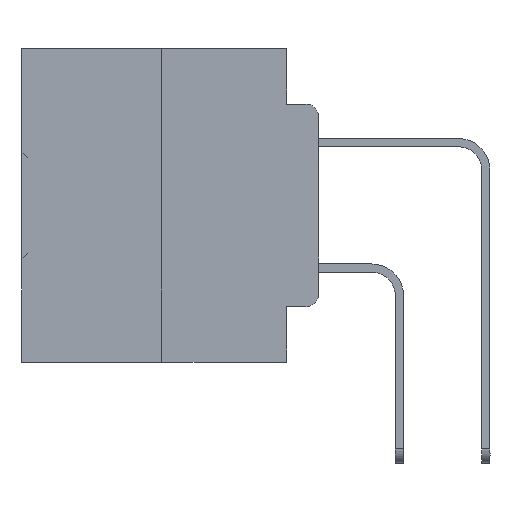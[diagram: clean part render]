
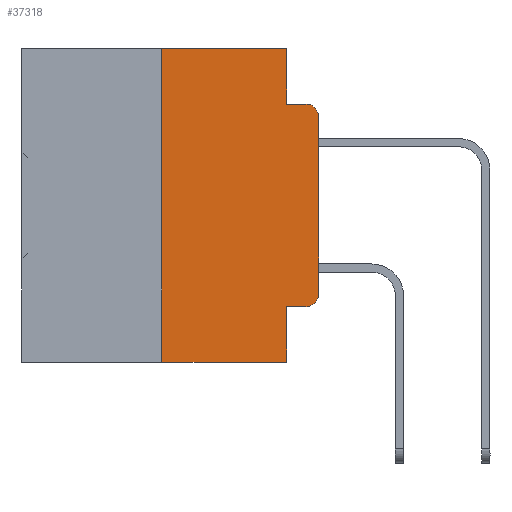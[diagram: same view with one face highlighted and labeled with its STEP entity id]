
A CAD part, left-side view. The second image highlights one B-rep face of the part: STEP entity #37318.
In plain terms, the highlighted planar face has unit normal (-1, 0, 0).
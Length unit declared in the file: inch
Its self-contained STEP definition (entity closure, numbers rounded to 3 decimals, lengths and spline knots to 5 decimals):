
#82 = VECTOR ( 'NONE', #9847, 39.37008 ) ;
#551 = ORIENTED_EDGE ( 'NONE', *, *, #11898, .T. ) ;
#628 = EDGE_CURVE ( 'NONE', #20644, #21502, #16890, .T. ) ;
#808 = CARTESIAN_POINT ( 'NONE',  ( 0., 0.02, -0.1085 ) ) ;
#951 = LINE ( 'NONE', #18273, #17860 ) ;
#1814 = DIRECTION ( 'NONE',  ( 1., 0., 0. ) ) ;
#1868 = DIRECTION ( 'NONE',  ( -1., 0., 0. ) ) ;
#1884 = ORIENTED_EDGE ( 'NONE', *, *, #18203, .F. ) ;
#2410 = CARTESIAN_POINT ( 'NONE',  ( 0., 0.051, -0.0885 ) ) ;
#2689 = CARTESIAN_POINT ( 'NONE',  ( 0., 0., -0.1085 ) ) ;
#2822 = VERTEX_POINT ( 'NONE', #36640 ) ;
#3727 = DIRECTION ( 'NONE',  ( 0., 0., 1. ) ) ;
#3755 = ORIENTED_EDGE ( 'NONE', *, *, #29755, .T. ) ;
#4560 = CIRCLE ( 'NONE', #31012, 0.02 ) ;
#5077 = PLANE ( 'NONE',  #7299 ) ;
#5140 = VERTEX_POINT ( 'NONE', #25508 ) ;
#5277 = CARTESIAN_POINT ( 'NONE',  ( 0., 0.25, 0. ) ) ;
#5418 = CARTESIAN_POINT ( 'NONE',  ( 0., 0.051, -0.5 ) ) ;
#6315 = DIRECTION ( 'NONE',  ( 0., 0., 1. ) ) ;
#6320 = EDGE_CURVE ( 'NONE', #5140, #35433, #21499, .T. ) ;
#6361 = VERTEX_POINT ( 'NONE', #36731 ) ;
#7162 = CARTESIAN_POINT ( 'NONE',  ( 0., 0., -0.3915 ) ) ;
#7299 = AXIS2_PLACEMENT_3D ( 'NONE', #22225, #1814, #22422 ) ;
#8712 = LINE ( 'NONE', #11243, #31086 ) ;
#9847 = DIRECTION ( 'NONE',  ( 0., 0., -1. ) ) ;
#10690 = ORIENTED_EDGE ( 'NONE', *, *, #628, .F. ) ;
#11243 = CARTESIAN_POINT ( 'NONE',  ( 0., 0.051, 0. ) ) ;
#11898 = EDGE_CURVE ( 'NONE', #6361, #26939, #4560, .T. ) ;
#11979 = EDGE_LOOP ( 'NONE', ( #26717, #3755, #10690, #24689, #18427, #1884, #12658, #35704, #31187, #551 ) ) ;
#12164 = LINE ( 'NONE', #30253, #82 ) ;
#12210 = CARTESIAN_POINT ( 'NONE',  ( 0., 0., 0. ) ) ;
#12476 = VECTOR ( 'NONE', #3727, 39.37008 ) ;
#12658 = ORIENTED_EDGE ( 'NONE', *, *, #6320, .T. ) ;
#14358 = CIRCLE ( 'NONE', #14960, 0.02 ) ;
#14960 = AXIS2_PLACEMENT_3D ( 'NONE', #808, #15659, #27743 ) ;
#15659 = DIRECTION ( 'NONE',  ( -1., 0., 0. ) ) ;
#15766 = DIRECTION ( 'NONE',  ( 0., -1., 0. ) ) ;
#16890 = LINE ( 'NONE', #2410, #23775 ) ;
#17860 = VECTOR ( 'NONE', #6315, 39.37008 ) ;
#17915 = CARTESIAN_POINT ( 'NONE',  ( 0., 0.473, 0. ) ) ;
#17986 = LINE ( 'NONE', #12210, #12476 ) ;
#18203 = EDGE_CURVE ( 'NONE', #5140, #37351, #951, .T. ) ;
#18273 = CARTESIAN_POINT ( 'NONE',  ( 0., 0.25, 0. ) ) ;
#18427 = ORIENTED_EDGE ( 'NONE', *, *, #34308, .F. ) ;
#19069 = EDGE_CURVE ( 'NONE', #2822, #35433, #12164, .T. ) ;
#19721 = FACE_OUTER_BOUND ( 'NONE', #11979, .T. ) ;
#20644 = VERTEX_POINT ( 'NONE', #25969 ) ;
#21499 = LINE ( 'NONE', #30919, #33946 ) ;
#21502 = VERTEX_POINT ( 'NONE', #30156 ) ;
#21923 = EDGE_CURVE ( 'NONE', #26939, #25903, #17986, .T. ) ;
#22041 = LINE ( 'NONE', #28192, #34871 ) ;
#22225 = CARTESIAN_POINT ( 'NONE',  ( 0., 0.473, 0. ) ) ;
#22422 = DIRECTION ( 'NONE',  ( 0., 0., -1. ) ) ;
#22502 = VERTEX_POINT ( 'NONE', #35769 ) ;
#23028 = DIRECTION ( 'NONE',  ( 0., -1., 0. ) ) ;
#23354 = DIRECTION ( 'NONE',  ( 0., 0., -1. ) ) ;
#23775 = VECTOR ( 'NONE', #23028, 39.37008 ) ;
#24689 = ORIENTED_EDGE ( 'NONE', *, *, #33732, .F. ) ;
#25508 = CARTESIAN_POINT ( 'NONE',  ( 0., 0.25, -0.5 ) ) ;
#25903 = VERTEX_POINT ( 'NONE', #2689 ) ;
#25969 = CARTESIAN_POINT ( 'NONE',  ( 0., 0.051, -0.0885 ) ) ;
#26717 = ORIENTED_EDGE ( 'NONE', *, *, #21923, .T. ) ;
#26932 = LINE ( 'NONE', #17915, #27422 ) ;
#26939 = VERTEX_POINT ( 'NONE', #7162 ) ;
#27422 = VECTOR ( 'NONE', #35079, 39.37008 ) ;
#27743 = DIRECTION ( 'NONE',  ( 0., 0., -1. ) ) ;
#28192 = CARTESIAN_POINT ( 'NONE',  ( 0., 0.051, -0.4115 ) ) ;
#28242 = CARTESIAN_POINT ( 'NONE',  ( 0., 0.02, -0.3915 ) ) ;
#29755 = EDGE_CURVE ( 'NONE', #25903, #21502, #14358, .T. ) ;
#30156 = CARTESIAN_POINT ( 'NONE',  ( 0., 0.02, -0.0885 ) ) ;
#30253 = CARTESIAN_POINT ( 'NONE',  ( 0., 0.051, 0. ) ) ;
#30889 = DIRECTION ( 'NONE',  ( 0., -1., 0. ) ) ;
#30919 = CARTESIAN_POINT ( 'NONE',  ( 0., 0.473, -0.5 ) ) ;
#31012 = AXIS2_PLACEMENT_3D ( 'NONE', #28242, #1868, #36564 ) ;
#31086 = VECTOR ( 'NONE', #23354, 39.37008 ) ;
#31187 = ORIENTED_EDGE ( 'NONE', *, *, #34910, .T. ) ;
#33732 = EDGE_CURVE ( 'NONE', #22502, #20644, #8712, .T. ) ;
#33946 = VECTOR ( 'NONE', #15766, 39.37008 ) ;
#34308 = EDGE_CURVE ( 'NONE', #37351, #22502, #26932, .T. ) ;
#34871 = VECTOR ( 'NONE', #30889, 39.37008 ) ;
#34910 = EDGE_CURVE ( 'NONE', #2822, #6361, #22041, .T. ) ;
#35079 = DIRECTION ( 'NONE',  ( 0., -1., 0. ) ) ;
#35433 = VERTEX_POINT ( 'NONE', #5418 ) ;
#35704 = ORIENTED_EDGE ( 'NONE', *, *, #19069, .F. ) ;
#35769 = CARTESIAN_POINT ( 'NONE',  ( 0., 0.051, 0. ) ) ;
#36564 = DIRECTION ( 'NONE',  ( 0., 0., -1. ) ) ;
#36640 = CARTESIAN_POINT ( 'NONE',  ( 0., 0.051, -0.4115 ) ) ;
#36731 = CARTESIAN_POINT ( 'NONE',  ( 0., 0.02, -0.4115 ) ) ;
#37318 = ADVANCED_FACE ( 'NONE', ( #19721 ), #5077, .F. ) ;
#37351 = VERTEX_POINT ( 'NONE', #5277 ) ;
